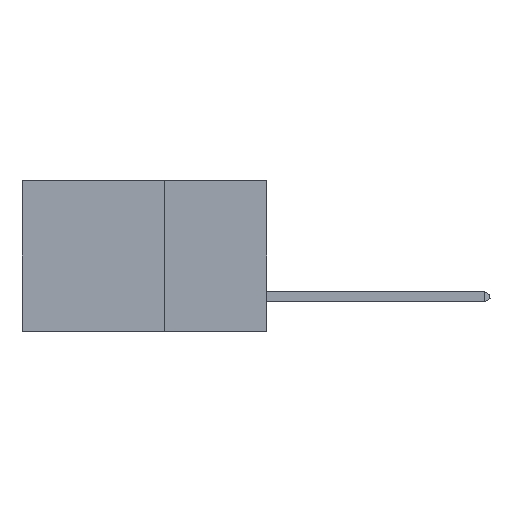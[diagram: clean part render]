
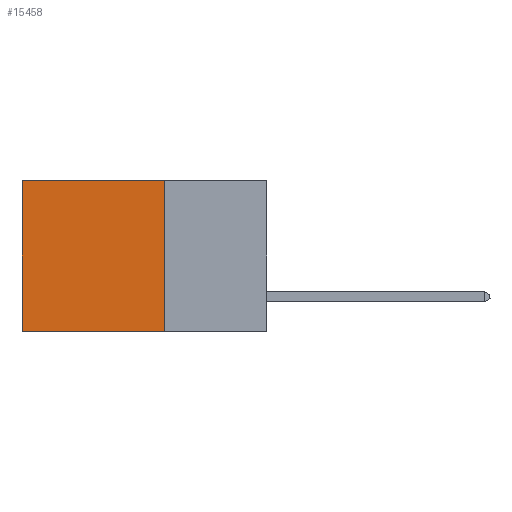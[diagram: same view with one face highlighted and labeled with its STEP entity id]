
A CAD part, left-side view. The second image highlights one B-rep face of the part: STEP entity #15458.
In plain terms, the highlighted planar face has unit normal (-1, 0, 0).
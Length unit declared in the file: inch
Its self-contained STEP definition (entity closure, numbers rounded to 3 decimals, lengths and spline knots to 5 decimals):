
#955 = DIRECTION ( 'NONE',  ( 0., 0., -1. ) ) ;
#2339 = ORIENTED_EDGE ( 'NONE', *, *, #10227, .F. ) ;
#2705 = AXIS2_PLACEMENT_3D ( 'NONE', #6992, #19276, #8812 ) ;
#2831 = CARTESIAN_POINT ( 'NONE',  ( 0.2875, 0.25, -0.37 ) ) ;
#3482 = CARTESIAN_POINT ( 'NONE',  ( 0.2875, 0.6, 0. ) ) ;
#5041 = LINE ( 'NONE', #6448, #8182 ) ;
#5291 = ORIENTED_EDGE ( 'NONE', *, *, #6462, .T. ) ;
#5313 = VERTEX_POINT ( 'NONE', #18208 ) ;
#6330 = EDGE_CURVE ( 'NONE', #5313, #8491, #14273, .T. ) ;
#6448 = CARTESIAN_POINT ( 'NONE',  ( 0.2875, 0.25, 0. ) ) ;
#6462 = EDGE_CURVE ( 'NONE', #9100, #5313, #7950, .T. ) ;
#6597 = CARTESIAN_POINT ( 'NONE',  ( 0.2875, 0.25, -0.37 ) ) ;
#6639 = VECTOR ( 'NONE', #10229, 39.37008 ) ;
#6729 = VERTEX_POINT ( 'NONE', #2831 ) ;
#6992 = CARTESIAN_POINT ( 'NONE',  ( 0.2875, 0.25, 0. ) ) ;
#7097 = VECTOR ( 'NONE', #7175, 39.37008 ) ;
#7175 = DIRECTION ( 'NONE',  ( 0., 0., -1. ) ) ;
#7950 = LINE ( 'NONE', #16432, #20262 ) ;
#8182 = VECTOR ( 'NONE', #955, 39.37008 ) ;
#8491 = VERTEX_POINT ( 'NONE', #20993 ) ;
#8812 = DIRECTION ( 'NONE',  ( 0., 0., -1. ) ) ;
#9100 = VERTEX_POINT ( 'NONE', #12491 ) ;
#10227 = EDGE_CURVE ( 'NONE', #6729, #8491, #16594, .T. ) ;
#10229 = DIRECTION ( 'NONE',  ( 0., 1., 0. ) ) ;
#11168 = FACE_OUTER_BOUND ( 'NONE', #17768, .T. ) ;
#12491 = CARTESIAN_POINT ( 'NONE',  ( 0.2875, 0.25, 0. ) ) ;
#14273 = LINE ( 'NONE', #3482, #7097 ) ;
#15458 = ADVANCED_FACE ( 'NONE', ( #11168 ), #20928, .F. ) ;
#15533 = ORIENTED_EDGE ( 'NONE', *, *, #20813, .F. ) ;
#15993 = ORIENTED_EDGE ( 'NONE', *, *, #6330, .T. ) ;
#16432 = CARTESIAN_POINT ( 'NONE',  ( 0.2875, 0.25, 0. ) ) ;
#16594 = LINE ( 'NONE', #6597, #6639 ) ;
#17768 = EDGE_LOOP ( 'NONE', ( #15993, #2339, #15533, #5291 ) ) ;
#18162 = DIRECTION ( 'NONE',  ( 0., 1., 0. ) ) ;
#18208 = CARTESIAN_POINT ( 'NONE',  ( 0.2875, 0.6, 0. ) ) ;
#19276 = DIRECTION ( 'NONE',  ( 1., 0., 0. ) ) ;
#20262 = VECTOR ( 'NONE', #18162, 39.37008 ) ;
#20813 = EDGE_CURVE ( 'NONE', #9100, #6729, #5041, .T. ) ;
#20928 = PLANE ( 'NONE',  #2705 ) ;
#20993 = CARTESIAN_POINT ( 'NONE',  ( 0.2875, 0.6, -0.37 ) ) ;
